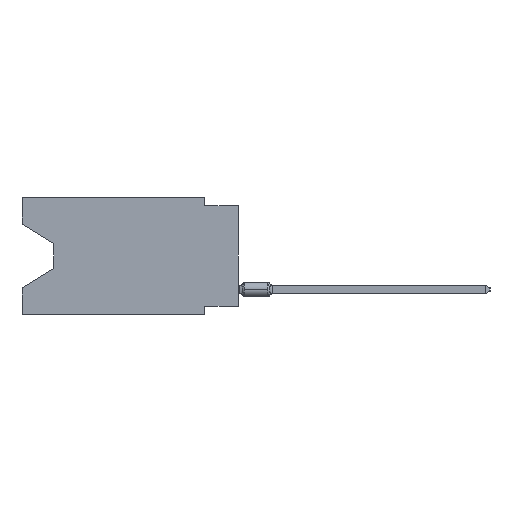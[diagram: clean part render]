
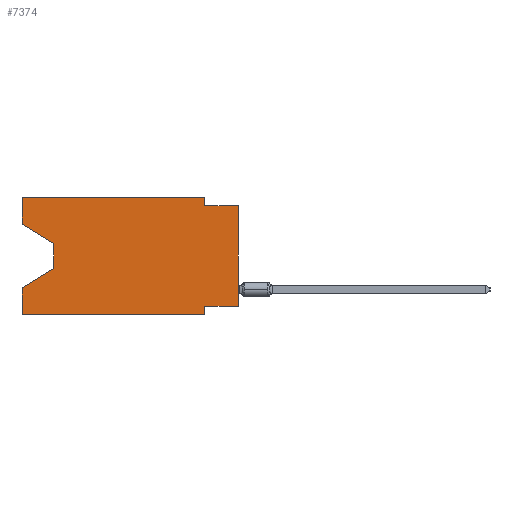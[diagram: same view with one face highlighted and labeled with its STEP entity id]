
A CAD part, left-side view. The second image highlights one B-rep face of the part: STEP entity #7374.
In plain terms, the highlighted planar face has unit normal (-1, 0, 0).
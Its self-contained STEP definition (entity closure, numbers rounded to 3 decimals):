
#69 = LINE ( 'NONE', #54449, #7856 ) ;
#303 = ORIENTED_EDGE ( 'NONE', *, *, #19622, .F. ) ;
#356 = CARTESIAN_POINT ( 'NONE',  ( 0., 16.383, -6.852 ) ) ;
#1169 = ORIENTED_EDGE ( 'NONE', *, *, #40258, .F. ) ;
#1801 = CARTESIAN_POINT ( 'NONE',  ( 0., 0., -8.255 ) ) ;
#2066 = DIRECTION ( 'NONE',  ( 0., -1., 0. ) ) ;
#2087 = PLANE ( 'NONE',  #45245 ) ;
#2243 = VERTEX_POINT ( 'NONE', #51475 ) ;
#2644 = EDGE_LOOP ( 'NONE', ( #22372, #37448, #64388, #30544, #10293, #38263, #21281, #13976, #32116, #5268, #303, #1169 ) ) ;
#2890 = DIRECTION ( 'NONE',  ( 0., -1., 0. ) ) ;
#3466 = CARTESIAN_POINT ( 'NONE',  ( 0., 0., -0.635 ) ) ;
#3707 = CARTESIAN_POINT ( 'NONE',  ( 0., 2.54, 0. ) ) ;
#4767 = CARTESIAN_POINT ( 'NONE',  ( 0., 16.383, 0. ) ) ;
#5268 = ORIENTED_EDGE ( 'NONE', *, *, #20723, .F. ) ;
#5475 = VECTOR ( 'NONE', #31251, 1000. ) ;
#6233 = LINE ( 'NONE', #66655, #31715 ) ;
#7064 = EDGE_CURVE ( 'NONE', #57271, #18616, #15374, .T. ) ;
#7374 = ADVANCED_FACE ( 'NONE', ( #66845 ), #2087, .F. ) ;
#7635 = VERTEX_POINT ( 'NONE', #59637 ) ;
#7856 = VECTOR ( 'NONE', #37293, 1000. ) ;
#8239 = VECTOR ( 'NONE', #58142, 1000. ) ;
#9667 = DIRECTION ( 'NONE',  ( 0., 0., 1. ) ) ;
#9989 = VECTOR ( 'NONE', #70749, 1000. ) ;
#9997 = CARTESIAN_POINT ( 'NONE',  ( 0., 16.383, -2.038 ) ) ;
#10005 = CARTESIAN_POINT ( 'NONE',  ( 0., 16.383, 0. ) ) ;
#10028 = CARTESIAN_POINT ( 'NONE',  ( 0., 0., 0. ) ) ;
#10077 = EDGE_CURVE ( 'NONE', #26531, #52540, #6233, .T. ) ;
#10293 = ORIENTED_EDGE ( 'NONE', *, *, #14745, .T. ) ;
#10790 = VECTOR ( 'NONE', #2066, 1000. ) ;
#12028 = EDGE_CURVE ( 'NONE', #68800, #61878, #69, .T. ) ;
#13976 = ORIENTED_EDGE ( 'NONE', *, *, #7064, .T. ) ;
#14745 = EDGE_CURVE ( 'NONE', #2243, #52540, #65070, .T. ) ;
#15374 = LINE ( 'NONE', #10028, #17770 ) ;
#16162 = VECTOR ( 'NONE', #37547, 1000. ) ;
#17770 = VECTOR ( 'NONE', #9667, 1000. ) ;
#18089 = CARTESIAN_POINT ( 'NONE',  ( 0., 2.54, 0. ) ) ;
#18522 = CARTESIAN_POINT ( 'NONE',  ( 0., 16.383, 0. ) ) ;
#18616 = VERTEX_POINT ( 'NONE', #3466 ) ;
#19226 = CARTESIAN_POINT ( 'NONE',  ( 0., 2.54, -8.255 ) ) ;
#19622 = EDGE_CURVE ( 'NONE', #23878, #54826, #33579, .T. ) ;
#20569 = CARTESIAN_POINT ( 'NONE',  ( 0., 16.383, 0. ) ) ;
#20723 = EDGE_CURVE ( 'NONE', #54826, #7635, #39214, .T. ) ;
#20753 = CARTESIAN_POINT ( 'NONE',  ( 0., 2.54, -8.89 ) ) ;
#21281 = ORIENTED_EDGE ( 'NONE', *, *, #68178, .F. ) ;
#22110 = CARTESIAN_POINT ( 'NONE',  ( 0., 0., -8.255 ) ) ;
#22372 = ORIENTED_EDGE ( 'NONE', *, *, #22644, .T. ) ;
#22644 = EDGE_CURVE ( 'NONE', #26713, #68800, #70058, .T. ) ;
#23878 = VERTEX_POINT ( 'NONE', #10005 ) ;
#23916 = DIRECTION ( 'NONE',  ( 0., 0., -1. ) ) ;
#25905 = DIRECTION ( 'NONE',  ( 0., 0., 1. ) ) ;
#26458 = CARTESIAN_POINT ( 'NONE',  ( 0., 16.383, -8.89 ) ) ;
#26531 = VERTEX_POINT ( 'NONE', #19226 ) ;
#26713 = VERTEX_POINT ( 'NONE', #64960 ) ;
#30544 = ORIENTED_EDGE ( 'NONE', *, *, #61404, .F. ) ;
#31251 = DIRECTION ( 'NONE',  ( 0., 0.855, -0.519 ) ) ;
#31715 = VECTOR ( 'NONE', #38791, 1000. ) ;
#32116 = ORIENTED_EDGE ( 'NONE', *, *, #62213, .F. ) ;
#33548 = VECTOR ( 'NONE', #2890, 1000. ) ;
#33579 = LINE ( 'NONE', #18522, #10790 ) ;
#35793 = LINE ( 'NONE', #52609, #33548 ) ;
#36326 = LINE ( 'NONE', #20569, #8239 ) ;
#36452 = VECTOR ( 'NONE', #53625, 1000. ) ;
#37161 = VERTEX_POINT ( 'NONE', #356 ) ;
#37293 = DIRECTION ( 'NONE',  ( 0., 0., -1. ) ) ;
#37448 = ORIENTED_EDGE ( 'NONE', *, *, #12028, .T. ) ;
#37547 = DIRECTION ( 'NONE',  ( 0., -1., 0. ) ) ;
#38263 = ORIENTED_EDGE ( 'NONE', *, *, #10077, .F. ) ;
#38791 = DIRECTION ( 'NONE',  ( 0., 0., -1. ) ) ;
#39214 = LINE ( 'NONE', #18089, #48573 ) ;
#39486 = VECTOR ( 'NONE', #25905, 1000. ) ;
#40258 = EDGE_CURVE ( 'NONE', #26713, #23878, #68797, .T. ) ;
#42325 = LINE ( 'NONE', #53761, #5475 ) ;
#43576 = LINE ( 'NONE', #22110, #9989 ) ;
#44691 = CARTESIAN_POINT ( 'NONE',  ( 0., 16.383, 0. ) ) ;
#45245 = AXIS2_PLACEMENT_3D ( 'NONE', #44691, #45392, #23916 ) ;
#45392 = DIRECTION ( 'NONE',  ( 1., 0., 0. ) ) ;
#48573 = VECTOR ( 'NONE', #62056, 1000. ) ;
#51475 = CARTESIAN_POINT ( 'NONE',  ( 0., 16.383, -8.89 ) ) ;
#52540 = VERTEX_POINT ( 'NONE', #20753 ) ;
#52609 = CARTESIAN_POINT ( 'NONE',  ( 0., 0., -0.635 ) ) ;
#53625 = DIRECTION ( 'NONE',  ( 0., -0.855, -0.519 ) ) ;
#53761 = CARTESIAN_POINT ( 'NONE',  ( 0., 13.97, -5.385 ) ) ;
#54449 = CARTESIAN_POINT ( 'NONE',  ( 0., 13.97, -3.505 ) ) ;
#54826 = VERTEX_POINT ( 'NONE', #3707 ) ;
#57271 = VERTEX_POINT ( 'NONE', #1801 ) ;
#58142 = DIRECTION ( 'NONE',  ( 0., 0., 1. ) ) ;
#59637 = CARTESIAN_POINT ( 'NONE',  ( 0., 2.54, -0.635 ) ) ;
#59761 = CARTESIAN_POINT ( 'NONE',  ( 0., 13.97, -3.505 ) ) ;
#61404 = EDGE_CURVE ( 'NONE', #2243, #37161, #36326, .T. ) ;
#61878 = VERTEX_POINT ( 'NONE', #65883 ) ;
#62056 = DIRECTION ( 'NONE',  ( 0., 0., -1. ) ) ;
#62213 = EDGE_CURVE ( 'NONE', #7635, #18616, #35793, .T. ) ;
#64388 = ORIENTED_EDGE ( 'NONE', *, *, #67117, .T. ) ;
#64960 = CARTESIAN_POINT ( 'NONE',  ( 0., 16.383, -2.038 ) ) ;
#65070 = LINE ( 'NONE', #26458, #16162 ) ;
#65883 = CARTESIAN_POINT ( 'NONE',  ( 0., 13.97, -5.385 ) ) ;
#66655 = CARTESIAN_POINT ( 'NONE',  ( 0., 2.54, -8.89 ) ) ;
#66845 = FACE_OUTER_BOUND ( 'NONE', #2644, .T. ) ;
#67117 = EDGE_CURVE ( 'NONE', #61878, #37161, #42325, .T. ) ;
#68178 = EDGE_CURVE ( 'NONE', #57271, #26531, #43576, .T. ) ;
#68797 = LINE ( 'NONE', #4767, #39486 ) ;
#68800 = VERTEX_POINT ( 'NONE', #59761 ) ;
#70058 = LINE ( 'NONE', #9997, #36452 ) ;
#70749 = DIRECTION ( 'NONE',  ( 0., 1., 0. ) ) ;
